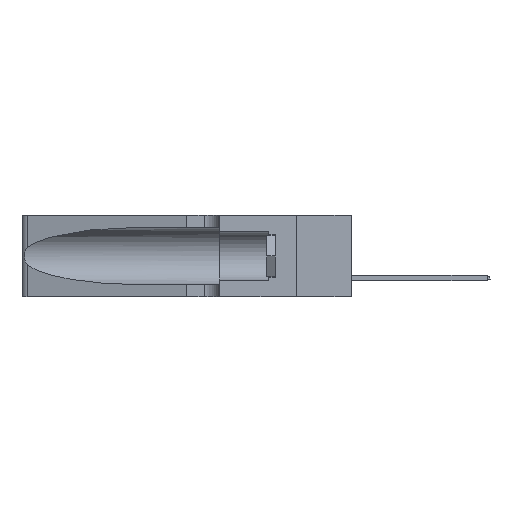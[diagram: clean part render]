
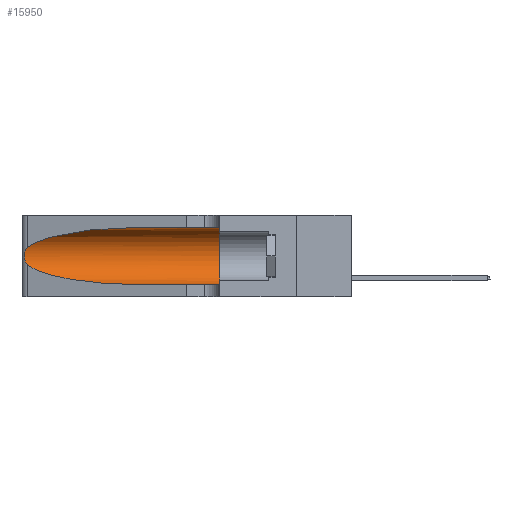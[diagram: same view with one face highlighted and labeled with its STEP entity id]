
A CAD part, left-side view. The second image highlights one B-rep face of the part: STEP entity #15950.
In plain terms, the highlighted cylindrical face has radius 3.308 mm (diameter 6.617 mm), a partial arc.
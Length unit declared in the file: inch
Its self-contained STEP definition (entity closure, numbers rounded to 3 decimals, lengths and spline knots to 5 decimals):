
#874 = AXIS2_PLACEMENT_3D ( 'NONE', #12112, #8636, #4974 ) ;
#979 = VERTEX_POINT ( 'NONE', #9485 ) ;
#1071 = CARTESIAN_POINT ( 'NONE',  ( 0.25856, 1.23593, 0.16098 ) ) ;
#2658 = VECTOR ( 'NONE', #45878, 39.37008 ) ;
#3670 = CARTESIAN_POINT ( 'NONE',  ( 0.26018, 1.23835, 0.19895 ) ) ;
#3975 = CARTESIAN_POINT ( 'NONE',  ( 0.26075, 1.23896, 0.178 ) ) ;
#4889 = DIRECTION ( 'NONE',  ( 0., -1., 0. ) ) ;
#4974 = DIRECTION ( 'NONE',  ( 0., 0., 1. ) ) ;
#5060 = LINE ( 'NONE', #40106, #7517 ) ;
#5575 = CARTESIAN_POINT ( 'NONE',  ( 0.25789, 1.23486, 0.15765 ) ) ;
#7517 = VECTOR ( 'NONE', #45824, 39.37008 ) ;
#7968 = LINE ( 'NONE', #26458, #2658 ) ;
#8048 = VERTEX_POINT ( 'NONE', #18715 ) ;
#8192 = EDGE_CURVE ( 'NONE', #979, #44902, #47494, .T. ) ;
#8467 = EDGE_CURVE ( 'NONE', #23556, #979, #20045, .T. ) ;
#8636 = DIRECTION ( 'NONE',  ( 0., 1., 0. ) ) ;
#9048 = CARTESIAN_POINT ( 'NONE',  ( 0.18966, 0.96281, 0.05475 ) ) ;
#9485 = CARTESIAN_POINT ( 'NONE',  ( 0.25487, 1.22718, 0.14631 ) ) ;
#10827 = CARTESIAN_POINT ( 'NONE',  ( 0.2373, 1.15595, 0.28018 ) ) ;
#12112 = CARTESIAN_POINT ( 'NONE',  ( 0.1305, 0.35, 0.185 ) ) ;
#14216 = ORIENTED_EDGE ( 'NONE', *, *, #16953, .F. ) ;
#15950 = ADVANCED_FACE ( 'NONE', ( #19461 ), #28343, .F. ) ;
#16659 = ORIENTED_EDGE ( 'NONE', *, *, #20238, .T. ) ;
#16687 = CARTESIAN_POINT ( 'NONE',  ( 0.1305, 0.72297, 0.05475 ) ) ;
#16953 = EDGE_CURVE ( 'NONE', #8048, #27353, #5060, .T. ) ;
#17261 = CARTESIAN_POINT ( 'NONE',  ( 0.25639, 1.23184, 0.21858 ) ) ;
#18311 = CARTESIAN_POINT ( 'NONE',  ( 0.18966, 0.96281, 0.31525 ) ) ;
#18715 = CARTESIAN_POINT ( 'NONE',  ( 0.1305, 0.72297, 0.31525 ) ) ;
#19016 = VERTEX_POINT ( 'NONE', #44012 ) ;
#19461 = FACE_OUTER_BOUND ( 'NONE', #23557, .T. ) ;
#20045 = B_SPLINE_CURVE_WITH_KNOTS ( 'NONE', 3,
 ( #38402, #28520, #17261, #22266, #22421, #3670, #41742, #3975, #30514, #1071, #5575, #24668, #44180, #22838 ),
 .UNSPECIFIED., .F., .F.,
 ( 4, 2, 2, 2, 2, 2, 4 ),
 ( 0., 0.00027, 0.00053, 0.00107, 0.0016, 0.00187, 0.00214 ),
 .UNSPECIFIED. ) ;
#20238 = EDGE_CURVE ( 'NONE', #8048, #23556, #37211, .T. ) ;
#21197 = CARTESIAN_POINT ( 'NONE',  ( 0.25487, 1.22718, 0.14631 ) ) ;
#22266 = CARTESIAN_POINT ( 'NONE',  ( 0.25787, 1.23484, 0.2124 ) ) ;
#22421 = CARTESIAN_POINT ( 'NONE',  ( 0.25854, 1.2359, 0.20912 ) ) ;
#22838 = CARTESIAN_POINT ( 'NONE',  ( 0.25487, 1.22718, 0.14631 ) ) ;
#23556 = VERTEX_POINT ( 'NONE', #32338 ) ;
#23557 = EDGE_LOOP ( 'NONE', ( #16659, #35151, #38874, #41632, #35647, #14216 ) ) ;
#24668 = CARTESIAN_POINT ( 'NONE',  ( 0.25639, 1.23186, 0.15144 ) ) ;
#24928 = CARTESIAN_POINT ( 'NONE',  ( 0.1305, 0.72297, 0.31525 ) ) ;
#25937 = AXIS2_PLACEMENT_3D ( 'NONE', #42976, #4889, #38969 ) ;
#26139 = CARTESIAN_POINT ( 'NONE',  ( 0.25487, 1.22718, 0.22369 ) ) ;
#26458 = CARTESIAN_POINT ( 'NONE',  ( 0.1305, 1.61858, 0.05475 ) ) ;
#27353 = VERTEX_POINT ( 'NONE', #40772 ) ;
#28343 = CYLINDRICAL_SURFACE ( 'NONE', #25937, 0.13025 ) ;
#28520 = CARTESIAN_POINT ( 'NONE',  ( 0.25555, 1.22994, 0.2215 ) ) ;
#30514 = CARTESIAN_POINT ( 'NONE',  ( 0.26017, 1.23833, 0.17102 ) ) ;
#32338 = CARTESIAN_POINT ( 'NONE',  ( 0.25487, 1.22718, 0.22369 ) ) ;
#33788 = EDGE_CURVE ( 'NONE', #27353, #19016, #47120, .T. ) ;
#35151 = ORIENTED_EDGE ( 'NONE', *, *, #8467, .T. ) ;
#35647 = ORIENTED_EDGE ( 'NONE', *, *, #33788, .F. ) ;
#37211 =( BOUNDED_CURVE ( )  B_SPLINE_CURVE ( 3, ( #24928, #18311, #10827, #26139 ),
 .UNSPECIFIED., .F., .F. ) 
 B_SPLINE_CURVE_WITH_KNOTS ( ( 4, 4 ),
 ( 1.5708, 2.84003 ),
 .UNSPECIFIED. ) 
 CURVE ( )  GEOMETRIC_REPRESENTATION_ITEM ( )  RATIONAL_B_SPLINE_CURVE ( ( 1., 0.87, 0.87, 1. ) ) 
 REPRESENTATION_ITEM ( '' )  );
#38402 = CARTESIAN_POINT ( 'NONE',  ( 0.25487, 1.22718, 0.22369 ) ) ;
#38807 = EDGE_CURVE ( 'NONE', #44902, #19016, #7968, .T. ) ;
#38874 = ORIENTED_EDGE ( 'NONE', *, *, #8192, .T. ) ;
#38969 = DIRECTION ( 'NONE',  ( 0., 0., -1. ) ) ;
#40106 = CARTESIAN_POINT ( 'NONE',  ( 0.1305, 1.61858, 0.31525 ) ) ;
#40772 = CARTESIAN_POINT ( 'NONE',  ( 0.1305, 0.35, 0.31525 ) ) ;
#41632 = ORIENTED_EDGE ( 'NONE', *, *, #38807, .T. ) ;
#41742 = CARTESIAN_POINT ( 'NONE',  ( 0.26075, 1.23896, 0.19203 ) ) ;
#42976 = CARTESIAN_POINT ( 'NONE',  ( 0.1305, 1.61858, 0.185 ) ) ;
#44012 = CARTESIAN_POINT ( 'NONE',  ( 0.1305, 0.35, 0.05475 ) ) ;
#44180 = CARTESIAN_POINT ( 'NONE',  ( 0.25555, 1.22993, 0.14849 ) ) ;
#44902 = VERTEX_POINT ( 'NONE', #49259 ) ;
#45824 = DIRECTION ( 'NONE',  ( 0., -1., 0. ) ) ;
#45878 = DIRECTION ( 'NONE',  ( 0., -1., 0. ) ) ;
#47120 = CIRCLE ( 'NONE', #874, 0.13025 ) ;
#47457 = CARTESIAN_POINT ( 'NONE',  ( 0.2373, 1.15595, 0.08982 ) ) ;
#47494 =( BOUNDED_CURVE ( )  B_SPLINE_CURVE ( 3, ( #21197, #47457, #9048, #16687 ),
 .UNSPECIFIED., .F., .F. ) 
 B_SPLINE_CURVE_WITH_KNOTS ( ( 4, 4 ),
 ( 3.44316, 4.71239 ),
 .UNSPECIFIED. ) 
 CURVE ( )  GEOMETRIC_REPRESENTATION_ITEM ( )  RATIONAL_B_SPLINE_CURVE ( ( 1., 0.87, 0.87, 1. ) ) 
 REPRESENTATION_ITEM ( '' )  );
#49259 = CARTESIAN_POINT ( 'NONE',  ( 0.1305, 0.72297, 0.05475 ) ) ;
